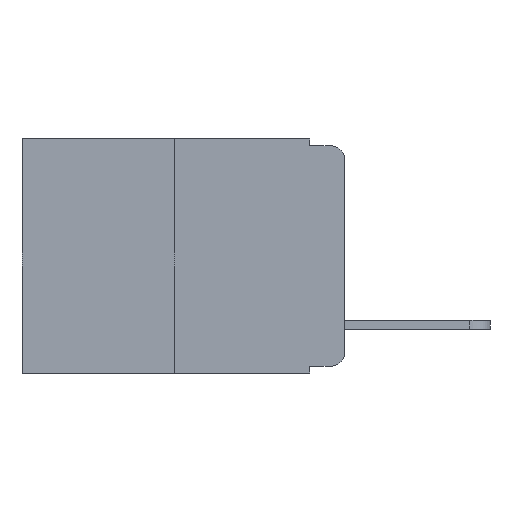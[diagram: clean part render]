
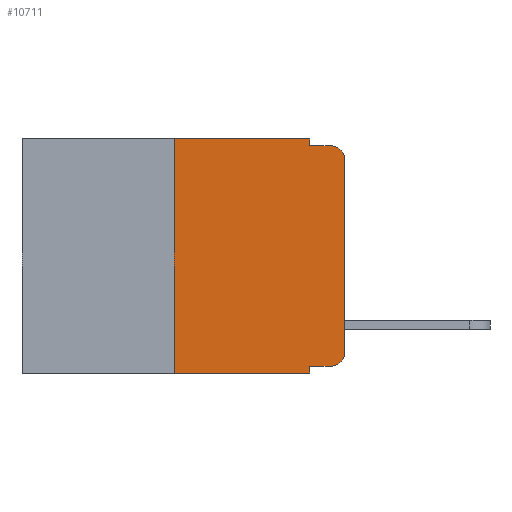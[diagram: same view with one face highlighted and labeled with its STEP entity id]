
A CAD part, left-side view. The second image highlights one B-rep face of the part: STEP entity #10711.
In plain terms, the highlighted planar face has unit normal (-1, 0, 0).
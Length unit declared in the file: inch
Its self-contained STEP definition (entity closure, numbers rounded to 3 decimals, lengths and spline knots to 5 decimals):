
#108 = VERTEX_POINT ( 'NONE', #15264 ) ;
#601 = DIRECTION ( 'NONE',  ( 0., 0., -1. ) ) ;
#907 = VERTEX_POINT ( 'NONE', #18485 ) ;
#1361 = VECTOR ( 'NONE', #9591, 39.37008 ) ;
#1364 = ORIENTED_EDGE ( 'NONE', *, *, #4906, .F. ) ;
#1624 = VECTOR ( 'NONE', #2041, 39.37008 ) ;
#1804 = DIRECTION ( 'NONE',  ( 0., 0., 1. ) ) ;
#1828 = VERTEX_POINT ( 'NONE', #11551 ) ;
#1983 = EDGE_CURVE ( 'NONE', #4171, #907, #14631, .T. ) ;
#2041 = DIRECTION ( 'NONE',  ( 0., 0., -1. ) ) ;
#2292 = CARTESIAN_POINT ( 'NONE',  ( 0., 0.473, 0. ) ) ;
#2441 = DIRECTION ( 'NONE',  ( 0., -1., 0. ) ) ;
#2518 = DIRECTION ( 'NONE',  ( 0., -1., 0. ) ) ;
#2750 = VERTEX_POINT ( 'NONE', #13881 ) ;
#2902 = CARTESIAN_POINT ( 'NONE',  ( 0., 0.02, -0.03 ) ) ;
#2963 = DIRECTION ( 'NONE',  ( -1., 0., 0. ) ) ;
#3247 = VECTOR ( 'NONE', #12823, 39.37008 ) ;
#3280 = DIRECTION ( 'NONE',  ( -1., 0., 0. ) ) ;
#3296 = AXIS2_PLACEMENT_3D ( 'NONE', #3299, #3280, #601 ) ;
#3299 = CARTESIAN_POINT ( 'NONE',  ( 0., 0.02, -0.313 ) ) ;
#3502 = DIRECTION ( 'NONE',  ( 0., 0., -1. ) ) ;
#3531 = CARTESIAN_POINT ( 'NONE',  ( 0., 0.25, -0.343 ) ) ;
#3542 = ORIENTED_EDGE ( 'NONE', *, *, #1983, .T. ) ;
#3600 = FACE_OUTER_BOUND ( 'NONE', #6587, .T. ) ;
#3682 = VECTOR ( 'NONE', #2518, 39.37008 ) ;
#3805 = VERTEX_POINT ( 'NONE', #17680 ) ;
#4054 = ORIENTED_EDGE ( 'NONE', *, *, #5023, .F. ) ;
#4171 = VERTEX_POINT ( 'NONE', #3531 ) ;
#4175 = VERTEX_POINT ( 'NONE', #12765 ) ;
#4299 = LINE ( 'NONE', #10995, #8047 ) ;
#4477 = EDGE_CURVE ( 'NONE', #108, #4520, #5816, .T. ) ;
#4520 = VERTEX_POINT ( 'NONE', #8831 ) ;
#4548 = LINE ( 'NONE', #14269, #12191 ) ;
#4570 = EDGE_CURVE ( 'NONE', #4520, #1828, #17863, .T. ) ;
#4811 = EDGE_CURVE ( 'NONE', #7498, #1828, #9930, .T. ) ;
#4906 = EDGE_CURVE ( 'NONE', #3805, #7498, #4299, .T. ) ;
#4931 = EDGE_CURVE ( 'NONE', #4171, #2750, #15578, .T. ) ;
#5023 = EDGE_CURVE ( 'NONE', #5560, #907, #13865, .T. ) ;
#5055 = EDGE_CURVE ( 'NONE', #5560, #4175, #4548, .T. ) ;
#5062 = CARTESIAN_POINT ( 'NONE',  ( 0., 0.473, -0.343 ) ) ;
#5153 = EDGE_CURVE ( 'NONE', #4175, #108, #10825, .T. ) ;
#5560 = VERTEX_POINT ( 'NONE', #12894 ) ;
#5816 = LINE ( 'NONE', #9432, #12858 ) ;
#6587 = EDGE_LOOP ( 'NONE', ( #15156, #19013, #9458, #1364, #9935, #14085, #3542, #4054, #12210, #8746 ) ) ;
#7088 = EDGE_CURVE ( 'NONE', #2750, #3805, #9348, .T. ) ;
#7140 = CARTESIAN_POINT ( 'NONE',  ( 0., 0.051, -0.01 ) ) ;
#7498 = VERTEX_POINT ( 'NONE', #17799 ) ;
#8047 = VECTOR ( 'NONE', #9276, 39.37008 ) ;
#8746 = ORIENTED_EDGE ( 'NONE', *, *, #5153, .T. ) ;
#8831 = CARTESIAN_POINT ( 'NONE',  ( 0., 0., -0.03 ) ) ;
#9276 = DIRECTION ( 'NONE',  ( 0., 0., -1. ) ) ;
#9348 = LINE ( 'NONE', #2292, #16294 ) ;
#9361 = CARTESIAN_POINT ( 'NONE',  ( 0., 0.25, 0. ) ) ;
#9396 = AXIS2_PLACEMENT_3D ( 'NONE', #2902, #2963, #3502 ) ;
#9432 = CARTESIAN_POINT ( 'NONE',  ( 0., 0., 0. ) ) ;
#9458 = ORIENTED_EDGE ( 'NONE', *, *, #4811, .F. ) ;
#9591 = DIRECTION ( 'NONE',  ( 0., -1., 0. ) ) ;
#9930 = LINE ( 'NONE', #7140, #1361 ) ;
#9935 = ORIENTED_EDGE ( 'NONE', *, *, #7088, .F. ) ;
#10711 = ADVANCED_FACE ( 'NONE', ( #3600 ), #15192, .F. ) ;
#10825 = CIRCLE ( 'NONE', #3296, 0.02 ) ;
#10954 = AXIS2_PLACEMENT_3D ( 'NONE', #15405, #15157, #15134 ) ;
#10995 = CARTESIAN_POINT ( 'NONE',  ( 0., 0.051, 0. ) ) ;
#11551 = CARTESIAN_POINT ( 'NONE',  ( 0., 0.02, -0.01 ) ) ;
#12191 = VECTOR ( 'NONE', #12916, 39.37008 ) ;
#12210 = ORIENTED_EDGE ( 'NONE', *, *, #5055, .T. ) ;
#12765 = CARTESIAN_POINT ( 'NONE',  ( 0., 0.02, -0.333 ) ) ;
#12823 = DIRECTION ( 'NONE',  ( 0., 0., 1. ) ) ;
#12858 = VECTOR ( 'NONE', #1804, 39.37008 ) ;
#12894 = CARTESIAN_POINT ( 'NONE',  ( 0., 0.051, -0.333 ) ) ;
#12916 = DIRECTION ( 'NONE',  ( 0., -1., 0. ) ) ;
#13865 = LINE ( 'NONE', #14076, #1624 ) ;
#13881 = CARTESIAN_POINT ( 'NONE',  ( 0., 0.25, 0. ) ) ;
#14076 = CARTESIAN_POINT ( 'NONE',  ( 0., 0.051, 0. ) ) ;
#14085 = ORIENTED_EDGE ( 'NONE', *, *, #4931, .F. ) ;
#14269 = CARTESIAN_POINT ( 'NONE',  ( 0., 0.051, -0.333 ) ) ;
#14631 = LINE ( 'NONE', #5062, #3682 ) ;
#15134 = DIRECTION ( 'NONE',  ( 0., 0., -1. ) ) ;
#15156 = ORIENTED_EDGE ( 'NONE', *, *, #4477, .T. ) ;
#15157 = DIRECTION ( 'NONE',  ( 1., 0., 0. ) ) ;
#15192 = PLANE ( 'NONE',  #10954 ) ;
#15264 = CARTESIAN_POINT ( 'NONE',  ( 0., 0., -0.313 ) ) ;
#15405 = CARTESIAN_POINT ( 'NONE',  ( 0., 0.473, 0. ) ) ;
#15578 = LINE ( 'NONE', #9361, #3247 ) ;
#16294 = VECTOR ( 'NONE', #2441, 39.37008 ) ;
#17680 = CARTESIAN_POINT ( 'NONE',  ( 0., 0.051, 0. ) ) ;
#17799 = CARTESIAN_POINT ( 'NONE',  ( 0., 0.051, -0.01 ) ) ;
#17863 = CIRCLE ( 'NONE', #9396, 0.02 ) ;
#18485 = CARTESIAN_POINT ( 'NONE',  ( 0., 0.051, -0.343 ) ) ;
#19013 = ORIENTED_EDGE ( 'NONE', *, *, #4570, .T. ) ;
